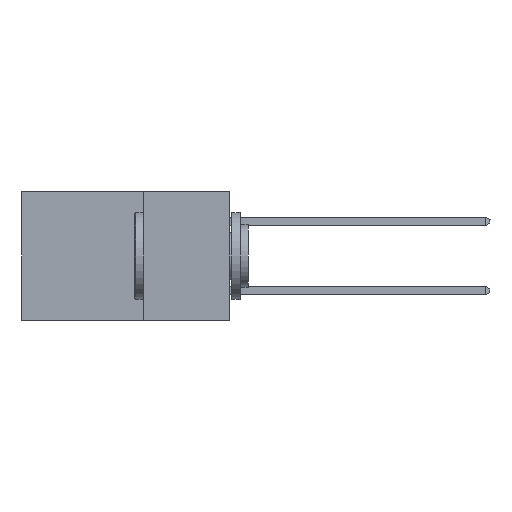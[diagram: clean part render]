
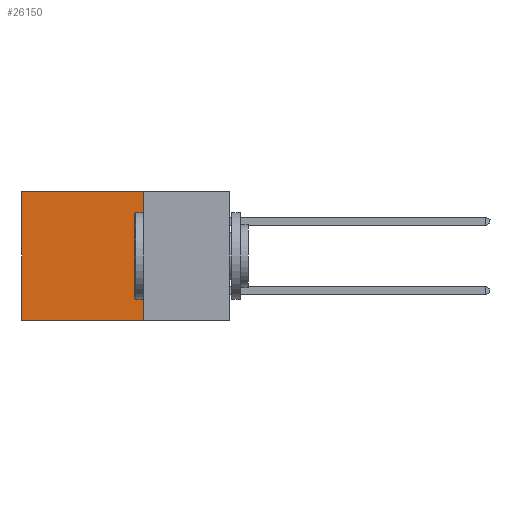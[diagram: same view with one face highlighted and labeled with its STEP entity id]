
A CAD part, left-side view. The second image highlights one B-rep face of the part: STEP entity #26150.
In plain terms, the highlighted planar face has unit normal (-1, 0, 0).
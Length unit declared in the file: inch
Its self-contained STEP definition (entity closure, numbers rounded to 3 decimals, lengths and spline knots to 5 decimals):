
#567 = CARTESIAN_POINT ( 'NONE',  ( 0.298, 0.6, 0. ) ) ;
#1098 = DIRECTION ( 'NONE',  ( 0., 1., 0. ) ) ;
#2132 = VERTEX_POINT ( 'NONE', #16875 ) ;
#2320 = CARTESIAN_POINT ( 'NONE',  ( 0.298, 0.6, 0. ) ) ;
#3644 = EDGE_LOOP ( 'NONE', ( #6343, #5130, #16777, #19430 ) ) ;
#4633 = EDGE_CURVE ( 'NONE', #5671, #26848, #19470, .T. ) ;
#5130 = ORIENTED_EDGE ( 'NONE', *, *, #25258, .F. ) ;
#5146 = LINE ( 'NONE', #18509, #28386 ) ;
#5671 = VERTEX_POINT ( 'NONE', #2320 ) ;
#6343 = ORIENTED_EDGE ( 'NONE', *, *, #4633, .T. ) ;
#6563 = CARTESIAN_POINT ( 'NONE',  ( 0.298, 0.6, -0.37 ) ) ;
#6920 = DIRECTION ( 'NONE',  ( 0., 1., 0. ) ) ;
#9913 = LINE ( 'NONE', #14786, #12446 ) ;
#10447 = LINE ( 'NONE', #28865, #22036 ) ;
#11973 = EDGE_CURVE ( 'NONE', #20715, #2132, #9913, .T. ) ;
#12199 = FACE_OUTER_BOUND ( 'NONE', #3644, .T. ) ;
#12446 = VECTOR ( 'NONE', #19476, 39.37008 ) ;
#14786 = CARTESIAN_POINT ( 'NONE',  ( 0.298, 0.25, 0. ) ) ;
#16777 = ORIENTED_EDGE ( 'NONE', *, *, #11973, .F. ) ;
#16835 = DIRECTION ( 'NONE',  ( 1., 0., 0. ) ) ;
#16875 = CARTESIAN_POINT ( 'NONE',  ( 0.298, 0.25, -0.37 ) ) ;
#17631 = VECTOR ( 'NONE', #23857, 39.37008 ) ;
#18509 = CARTESIAN_POINT ( 'NONE',  ( 0.298, 0.25, 0. ) ) ;
#18976 = PLANE ( 'NONE',  #22955 ) ;
#19430 = ORIENTED_EDGE ( 'NONE', *, *, #22639, .T. ) ;
#19470 = LINE ( 'NONE', #567, #17631 ) ;
#19476 = DIRECTION ( 'NONE',  ( 0., 0., -1. ) ) ;
#20715 = VERTEX_POINT ( 'NONE', #27708 ) ;
#21588 = DIRECTION ( 'NONE',  ( 0., 0., -1. ) ) ;
#22036 = VECTOR ( 'NONE', #1098, 39.37008 ) ;
#22639 = EDGE_CURVE ( 'NONE', #20715, #5671, #5146, .T. ) ;
#22955 = AXIS2_PLACEMENT_3D ( 'NONE', #26001, #16835, #21588 ) ;
#23857 = DIRECTION ( 'NONE',  ( 0., 0., -1. ) ) ;
#25258 = EDGE_CURVE ( 'NONE', #2132, #26848, #10447, .T. ) ;
#26001 = CARTESIAN_POINT ( 'NONE',  ( 0.298, 0.25, 0. ) ) ;
#26150 = ADVANCED_FACE ( 'NONE', ( #12199 ), #18976, .F. ) ;
#26848 = VERTEX_POINT ( 'NONE', #6563 ) ;
#27708 = CARTESIAN_POINT ( 'NONE',  ( 0.298, 0.25, 0. ) ) ;
#28386 = VECTOR ( 'NONE', #6920, 39.37008 ) ;
#28865 = CARTESIAN_POINT ( 'NONE',  ( 0.298, 0.25, -0.37 ) ) ;
